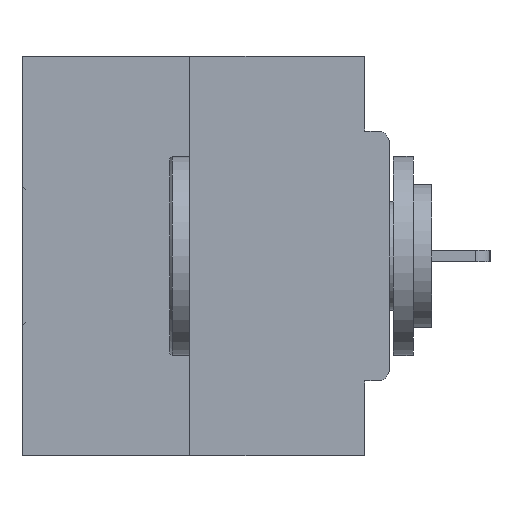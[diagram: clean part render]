
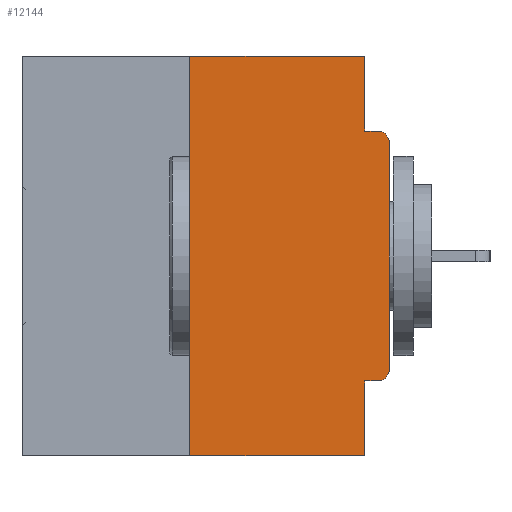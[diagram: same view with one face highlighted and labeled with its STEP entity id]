
A CAD part, left-side view. The second image highlights one B-rep face of the part: STEP entity #12144.
In plain terms, the highlighted planar face has unit normal (-1, 0, 0).
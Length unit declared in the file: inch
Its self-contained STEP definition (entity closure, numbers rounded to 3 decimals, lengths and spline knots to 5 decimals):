
#792 = DIRECTION ( 'NONE',  ( 0., -1., 0. ) ) ;
#861 = PLANE ( 'NONE',  #19812 ) ;
#921 = CARTESIAN_POINT ( 'NONE',  ( 0., 0.015, -0.1085 ) ) ;
#1118 = DIRECTION ( 'NONE',  ( 0., 0., -1. ) ) ;
#1211 = DIRECTION ( 'NONE',  ( 0., -1., 0. ) ) ;
#1255 = CARTESIAN_POINT ( 'NONE',  ( 0., 0.25, 0. ) ) ;
#1621 = VERTEX_POINT ( 'NONE', #20190 ) ;
#1978 = EDGE_CURVE ( 'NONE', #11556, #16471, #4136, .T. ) ;
#2722 = VERTEX_POINT ( 'NONE', #21958 ) ;
#3170 = DIRECTION ( 'NONE',  ( -1., 0., 0. ) ) ;
#3287 = VECTOR ( 'NONE', #21908, 39.37008 ) ;
#3460 = CARTESIAN_POINT ( 'NONE',  ( 0., 0.25, -0.5 ) ) ;
#3503 = CARTESIAN_POINT ( 'NONE',  ( 0., 0., -0.0935 ) ) ;
#4136 = LINE ( 'NONE', #6999, #28244 ) ;
#4449 = EDGE_CURVE ( 'NONE', #16471, #7531, #16460, .T. ) ;
#4712 = DIRECTION ( 'NONE',  ( -1., 0., 0. ) ) ;
#5079 = EDGE_CURVE ( 'NONE', #9916, #31340, #17219, .T. ) ;
#6010 = LINE ( 'NONE', #3503, #28496 ) ;
#6999 = CARTESIAN_POINT ( 'NONE',  ( 0., 0., 0. ) ) ;
#7100 = EDGE_LOOP ( 'NONE', ( #27819, #29469, #17689, #32716, #17686, #18415, #19490, #10001, #14046, #8072 ) ) ;
#7334 = CARTESIAN_POINT ( 'NONE',  ( 0., 0.46, 0. ) ) ;
#7531 = VERTEX_POINT ( 'NONE', #9028 ) ;
#8072 = ORIENTED_EDGE ( 'NONE', *, *, #27300, .F. ) ;
#8460 = CARTESIAN_POINT ( 'NONE',  ( 0., 0.46, -0.5 ) ) ;
#9028 = CARTESIAN_POINT ( 'NONE',  ( 0., 0.015, -0.0935 ) ) ;
#9700 = EDGE_CURVE ( 'NONE', #37575, #1621, #27384, .T. ) ;
#9916 = VERTEX_POINT ( 'NONE', #3460 ) ;
#10001 = ORIENTED_EDGE ( 'NONE', *, *, #4449, .T. ) ;
#10204 = LINE ( 'NONE', #7334, #14771 ) ;
#10218 = CARTESIAN_POINT ( 'NONE',  ( 0., 0., -0.1085 ) ) ;
#10232 = DIRECTION ( 'NONE',  ( 1., 0., 0. ) ) ;
#10986 = AXIS2_PLACEMENT_3D ( 'NONE', #921, #4712, #1118 ) ;
#11556 = VERTEX_POINT ( 'NONE', #34927 ) ;
#12144 = ADVANCED_FACE ( 'NONE', ( #27048 ), #861, .F. ) ;
#12321 = CARTESIAN_POINT ( 'NONE',  ( 0., 0.031, -0.5 ) ) ;
#12595 = VECTOR ( 'NONE', #17903, 39.37008 ) ;
#13628 = EDGE_CURVE ( 'NONE', #17184, #23982, #10204, .T. ) ;
#13819 = LINE ( 'NONE', #16674, #3287 ) ;
#14046 = ORIENTED_EDGE ( 'NONE', *, *, #20249, .F. ) ;
#14320 = VECTOR ( 'NONE', #27603, 39.37008 ) ;
#14771 = VECTOR ( 'NONE', #1211, 39.37008 ) ;
#15751 = DIRECTION ( 'NONE',  ( 0., 0., 1. ) ) ;
#16044 = CIRCLE ( 'NONE', #20972, 0.015 ) ;
#16056 = CARTESIAN_POINT ( 'NONE',  ( 0., 0., -0.4065 ) ) ;
#16460 = CIRCLE ( 'NONE', #10986, 0.015 ) ;
#16471 = VERTEX_POINT ( 'NONE', #10218 ) ;
#16674 = CARTESIAN_POINT ( 'NONE',  ( 0., 0.031, 0. ) ) ;
#17184 = VERTEX_POINT ( 'NONE', #1255 ) ;
#17219 = LINE ( 'NONE', #8460, #22664 ) ;
#17686 = ORIENTED_EDGE ( 'NONE', *, *, #9700, .F. ) ;
#17689 = ORIENTED_EDGE ( 'NONE', *, *, #5079, .T. ) ;
#17903 = DIRECTION ( 'NONE',  ( 0., 0., -1. ) ) ;
#18415 = ORIENTED_EDGE ( 'NONE', *, *, #26926, .T. ) ;
#19391 = EDGE_CURVE ( 'NONE', #1621, #31340, #26723, .T. ) ;
#19490 = ORIENTED_EDGE ( 'NONE', *, *, #1978, .T. ) ;
#19812 = AXIS2_PLACEMENT_3D ( 'NONE', #24961, #10232, #36028 ) ;
#20190 = CARTESIAN_POINT ( 'NONE',  ( 0., 0.031, -0.4065 ) ) ;
#20249 = EDGE_CURVE ( 'NONE', #2722, #7531, #6010, .T. ) ;
#20592 = CARTESIAN_POINT ( 'NONE',  ( 0., 0.031, 0. ) ) ;
#20972 = AXIS2_PLACEMENT_3D ( 'NONE', #31847, #3170, #35265 ) ;
#21186 = CARTESIAN_POINT ( 'NONE',  ( 0., 0.031, -0.5 ) ) ;
#21908 = DIRECTION ( 'NONE',  ( 0., 0., -1. ) ) ;
#21958 = CARTESIAN_POINT ( 'NONE',  ( 0., 0.031, -0.0935 ) ) ;
#22031 = DIRECTION ( 'NONE',  ( 0., 1., 0. ) ) ;
#22664 = VECTOR ( 'NONE', #28894, 39.37008 ) ;
#22828 = VECTOR ( 'NONE', #22031, 39.37008 ) ;
#23982 = VERTEX_POINT ( 'NONE', #20592 ) ;
#24961 = CARTESIAN_POINT ( 'NONE',  ( 0., 0.46, 0. ) ) ;
#26723 = LINE ( 'NONE', #21186, #12595 ) ;
#26926 = EDGE_CURVE ( 'NONE', #37575, #11556, #16044, .T. ) ;
#27048 = FACE_OUTER_BOUND ( 'NONE', #7100, .T. ) ;
#27300 = EDGE_CURVE ( 'NONE', #23982, #2722, #13819, .T. ) ;
#27384 = LINE ( 'NONE', #16056, #22828 ) ;
#27603 = DIRECTION ( 'NONE',  ( 0., 0., 1. ) ) ;
#27819 = ORIENTED_EDGE ( 'NONE', *, *, #13628, .F. ) ;
#28244 = VECTOR ( 'NONE', #15751, 39.37008 ) ;
#28496 = VECTOR ( 'NONE', #792, 39.37008 ) ;
#28894 = DIRECTION ( 'NONE',  ( 0., -1., 0. ) ) ;
#29469 = ORIENTED_EDGE ( 'NONE', *, *, #33711, .F. ) ;
#29771 = CARTESIAN_POINT ( 'NONE',  ( 0., 0.015, -0.4065 ) ) ;
#30469 = CARTESIAN_POINT ( 'NONE',  ( 0., 0.25, 0. ) ) ;
#31340 = VERTEX_POINT ( 'NONE', #12321 ) ;
#31847 = CARTESIAN_POINT ( 'NONE',  ( 0., 0.015, -0.3915 ) ) ;
#32716 = ORIENTED_EDGE ( 'NONE', *, *, #19391, .F. ) ;
#33339 = LINE ( 'NONE', #30469, #14320 ) ;
#33711 = EDGE_CURVE ( 'NONE', #9916, #17184, #33339, .T. ) ;
#34927 = CARTESIAN_POINT ( 'NONE',  ( 0., 0., -0.3915 ) ) ;
#35265 = DIRECTION ( 'NONE',  ( 0., 0., -1. ) ) ;
#36028 = DIRECTION ( 'NONE',  ( 0., 0., -1. ) ) ;
#37575 = VERTEX_POINT ( 'NONE', #29771 ) ;
